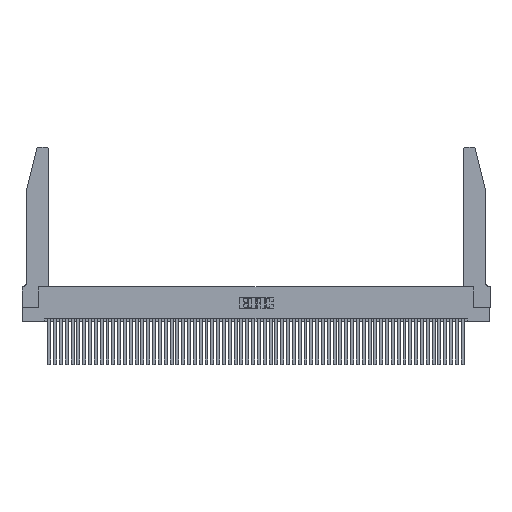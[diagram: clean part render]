
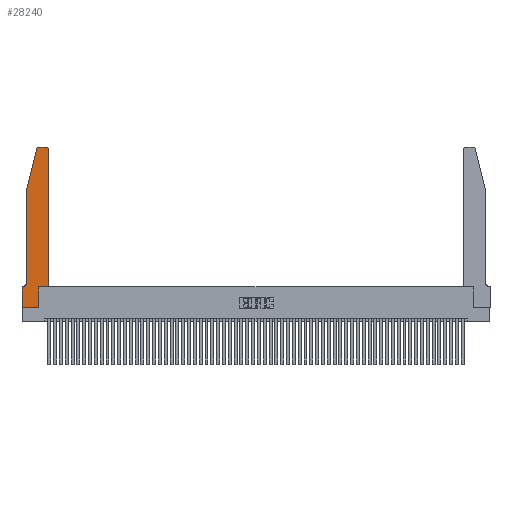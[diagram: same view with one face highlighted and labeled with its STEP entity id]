
A CAD part, top view. The second image highlights one B-rep face of the part: STEP entity #28240.
In plain terms, the highlighted planar face has unit normal (0, 0, 1).
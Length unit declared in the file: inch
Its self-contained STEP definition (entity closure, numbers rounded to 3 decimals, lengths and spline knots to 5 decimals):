
#765 = ORIENTED_EDGE ( 'NONE', *, *, #26465, .T. ) ;
#807 = PLANE ( 'NONE',  #1796 ) ;
#1629 = CARTESIAN_POINT ( 'NONE',  ( 0., 0., 0.37 ) ) ;
#1796 = AXIS2_PLACEMENT_3D ( 'NONE', #44958, #5322, #36412 ) ;
#2200 = CARTESIAN_POINT ( 'NONE',  ( 0., 0.35, 0.37 ) ) ;
#2541 = CARTESIAN_POINT ( 'NONE',  ( 0.0055, 0.42, 0.37 ) ) ;
#2605 = CARTESIAN_POINT ( 'NONE',  ( 0.2865, 0., 0.37 ) ) ;
#2683 = CIRCLE ( 'NONE', #6958, 0.07 ) ;
#2946 = CARTESIAN_POINT ( 'NONE',  ( 0.25487, 2.72718, 0.37 ) ) ;
#5251 = VERTEX_POINT ( 'NONE', #24601 ) ;
#5322 = DIRECTION ( 'NONE',  ( 0., 0., 1. ) ) ;
#6282 = VECTOR ( 'NONE', #6976, 39.37008 ) ;
#6958 = AXIS2_PLACEMENT_3D ( 'NONE', #2541, #33718, #7038 ) ;
#6976 = DIRECTION ( 'NONE',  ( 0., 1., 0. ) ) ;
#7038 = DIRECTION ( 'NONE',  ( -1., 0., 0. ) ) ;
#8820 = VERTEX_POINT ( 'NONE', #27613 ) ;
#9700 = LINE ( 'NONE', #51086, #55068 ) ;
#10415 = CARTESIAN_POINT ( 'NONE',  ( 0., 0., 0.37 ) ) ;
#10761 = CARTESIAN_POINT ( 'NONE',  ( 0.2865, 0.35, 0.37 ) ) ;
#13444 = ORIENTED_EDGE ( 'NONE', *, *, #32222, .T. ) ;
#13505 = ORIENTED_EDGE ( 'NONE', *, *, #16861, .T. ) ;
#13572 = CARTESIAN_POINT ( 'NONE',  ( 0.0755, 2., 0.37 ) ) ;
#13990 = CARTESIAN_POINT ( 'NONE',  ( 0.284, 2.75, 0.37 ) ) ;
#14980 = DIRECTION ( 'NONE',  ( 0., 0., 1. ) ) ;
#16174 = DIRECTION ( 'NONE',  ( -1., 0., 0. ) ) ;
#16474 = VECTOR ( 'NONE', #54409, 39.37008 ) ;
#16823 = ORIENTED_EDGE ( 'NONE', *, *, #56447, .T. ) ;
#16861 = EDGE_CURVE ( 'NONE', #8820, #50510, #9700, .T. ) ;
#17910 = VECTOR ( 'NONE', #46035, 39.37008 ) ;
#18045 = VECTOR ( 'NONE', #47838, 39.37008 ) ;
#18546 = LINE ( 'NONE', #22076, #30410 ) ;
#18731 = ORIENTED_EDGE ( 'NONE', *, *, #24844, .T. ) ;
#19195 = EDGE_CURVE ( 'NONE', #33414, #56409, #20859, .T. ) ;
#20495 = CARTESIAN_POINT ( 'NONE',  ( 0.0755, 2., 0.37 ) ) ;
#20859 = LINE ( 'NONE', #56538, #18045 ) ;
#22076 = CARTESIAN_POINT ( 'NONE',  ( 0., 0., 0.37 ) ) ;
#22112 = ORIENTED_EDGE ( 'NONE', *, *, #23365, .T. ) ;
#22492 = CARTESIAN_POINT ( 'NONE',  ( 0.4505, 0.35, 0.37 ) ) ;
#22626 = DIRECTION ( 'NONE',  ( -1., 0., 0. ) ) ;
#22939 = DIRECTION ( 'NONE',  ( 0., 0., 1. ) ) ;
#23365 = EDGE_CURVE ( 'NONE', #36432, #30369, #42335, .T. ) ;
#24601 = CARTESIAN_POINT ( 'NONE',  ( 0.0755, 0.42, 0.37 ) ) ;
#24654 = ORIENTED_EDGE ( 'NONE', *, *, #27726, .T. ) ;
#24844 = EDGE_CURVE ( 'NONE', #5251, #36432, #2683, .T. ) ;
#26465 = EDGE_CURVE ( 'NONE', #56889, #8820, #47593, .T. ) ;
#26642 = ORIENTED_EDGE ( 'NONE', *, *, #44259, .T. ) ;
#27613 = CARTESIAN_POINT ( 'NONE',  ( 0.4205, 2.75, 0.37 ) ) ;
#27726 = EDGE_CURVE ( 'NONE', #39136, #32257, #33897, .T. ) ;
#28240 = ADVANCED_FACE ( 'NONE', ( #39341 ), #807, .T. ) ;
#28348 = LINE ( 'NONE', #1629, #16474 ) ;
#28907 = EDGE_CURVE ( 'NONE', #32257, #44083, #51441, .T. ) ;
#29249 = CARTESIAN_POINT ( 'NONE',  ( 0.4505, 0.35, 0.37 ) ) ;
#30369 = VERTEX_POINT ( 'NONE', #2200 ) ;
#30410 = VECTOR ( 'NONE', #30996, 39.37008 ) ;
#30996 = DIRECTION ( 'NONE',  ( 0., -1., 0. ) ) ;
#31698 = CARTESIAN_POINT ( 'NONE',  ( 0.4505, 0.35, 0.37 ) ) ;
#32126 = AXIS2_PLACEMENT_3D ( 'NONE', #49091, #22939, #53453 ) ;
#32222 = EDGE_CURVE ( 'NONE', #30369, #33132, #18546, .T. ) ;
#32257 = VERTEX_POINT ( 'NONE', #56941 ) ;
#33132 = VERTEX_POINT ( 'NONE', #10415 ) ;
#33414 = VERTEX_POINT ( 'NONE', #2946 ) ;
#33718 = DIRECTION ( 'NONE',  ( 0., 0., -1. ) ) ;
#33897 = LINE ( 'NONE', #10761, #17910 ) ;
#36343 = EDGE_LOOP ( 'NONE', ( #13505, #16823, #42894, #37421, #18731, #22112, #13444, #26642, #24654, #45876, #50480, #765 ) ) ;
#36412 = DIRECTION ( 'NONE',  ( 1., 0., 0. ) ) ;
#36432 = VERTEX_POINT ( 'NONE', #44016 ) ;
#37421 = ORIENTED_EDGE ( 'NONE', *, *, #46718, .T. ) ;
#39136 = VERTEX_POINT ( 'NONE', #2605 ) ;
#39341 = FACE_OUTER_BOUND ( 'NONE', #36343, .T. ) ;
#39921 = VECTOR ( 'NONE', #40145, 39.37008 ) ;
#40145 = DIRECTION ( 'NONE',  ( 1., 0., 0. ) ) ;
#41422 = CARTESIAN_POINT ( 'NONE',  ( 0.4205, 2.72, 0.37 ) ) ;
#42335 = LINE ( 'NONE', #53148, #51139 ) ;
#42446 = VECTOR ( 'NONE', #55441, 39.37008 ) ;
#42894 = ORIENTED_EDGE ( 'NONE', *, *, #19195, .T. ) ;
#44016 = CARTESIAN_POINT ( 'NONE',  ( 0.0055, 0.35, 0.37 ) ) ;
#44083 = VERTEX_POINT ( 'NONE', #31698 ) ;
#44259 = EDGE_CURVE ( 'NONE', #33132, #39136, #28348, .T. ) ;
#44958 = CARTESIAN_POINT ( 'NONE',  ( 0., 0.35, 0.37 ) ) ;
#45771 = DIRECTION ( 'NONE',  ( 1., 0., 0. ) ) ;
#45876 = ORIENTED_EDGE ( 'NONE', *, *, #28907, .T. ) ;
#46035 = DIRECTION ( 'NONE',  ( 0., 1., 0. ) ) ;
#46718 = EDGE_CURVE ( 'NONE', #56409, #5251, #53953, .T. ) ;
#46929 = AXIS2_PLACEMENT_3D ( 'NONE', #41422, #14980, #45771 ) ;
#47593 = CIRCLE ( 'NONE', #46929, 0.03 ) ;
#47838 = DIRECTION ( 'NONE',  ( -0.239, -0.971, 0. ) ) ;
#49091 = CARTESIAN_POINT ( 'NONE',  ( 0.284, 2.72, 0.37 ) ) ;
#50480 = ORIENTED_EDGE ( 'NONE', *, *, #52179, .T. ) ;
#50510 = VERTEX_POINT ( 'NONE', #13990 ) ;
#51086 = CARTESIAN_POINT ( 'NONE',  ( 0.2605, 2.75, 0.37 ) ) ;
#51139 = VECTOR ( 'NONE', #22626, 39.37008 ) ;
#51322 = CIRCLE ( 'NONE', #32126, 0.03 ) ;
#51441 = LINE ( 'NONE', #22492, #39921 ) ;
#52179 = EDGE_CURVE ( 'NONE', #44083, #56889, #53092, .T. ) ;
#53092 = LINE ( 'NONE', #29249, #6282 ) ;
#53148 = CARTESIAN_POINT ( 'NONE',  ( 0.0755, 0.35, 0.37 ) ) ;
#53453 = DIRECTION ( 'NONE',  ( 1., 0., 0. ) ) ;
#53953 = LINE ( 'NONE', #20495, #42446 ) ;
#54409 = DIRECTION ( 'NONE',  ( 1., 0., 0. ) ) ;
#55068 = VECTOR ( 'NONE', #16174, 39.37008 ) ;
#55441 = DIRECTION ( 'NONE',  ( 0., -1., 0. ) ) ;
#56063 = CARTESIAN_POINT ( 'NONE',  ( 0.4505, 2.72, 0.37 ) ) ;
#56409 = VERTEX_POINT ( 'NONE', #13572 ) ;
#56447 = EDGE_CURVE ( 'NONE', #50510, #33414, #51322, .T. ) ;
#56538 = CARTESIAN_POINT ( 'NONE',  ( 0.0755, 2., 0.37 ) ) ;
#56889 = VERTEX_POINT ( 'NONE', #56063 ) ;
#56941 = CARTESIAN_POINT ( 'NONE',  ( 0.2865, 0.35, 0.37 ) ) ;
